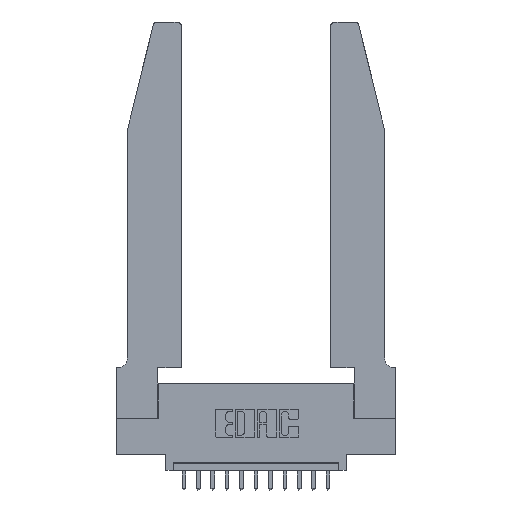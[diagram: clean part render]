
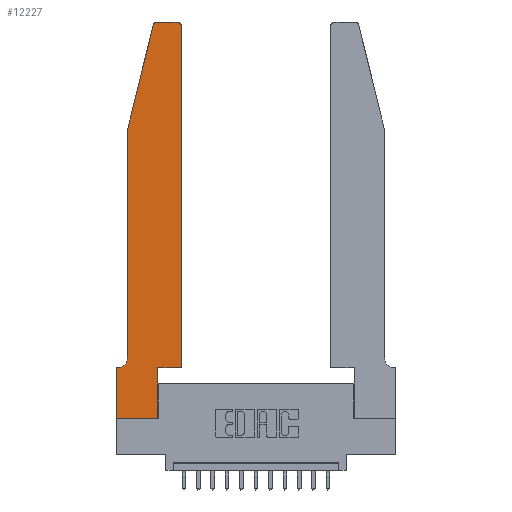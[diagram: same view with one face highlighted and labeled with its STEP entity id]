
A CAD part, top view. The second image highlights one B-rep face of the part: STEP entity #12227.
In plain terms, the highlighted planar face has unit normal (0, 0, 1).
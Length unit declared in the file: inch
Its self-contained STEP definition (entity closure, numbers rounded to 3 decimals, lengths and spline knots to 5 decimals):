
#383 = DIRECTION ( 'NONE',  ( -0.239, -0.971, 0. ) ) ;
#654 = VECTOR ( 'NONE', #7772, 39.37008 ) ;
#697 = VERTEX_POINT ( 'NONE', #13475 ) ;
#800 = EDGE_CURVE ( 'NONE', #697, #3935, #15390, .T. ) ;
#808 = CARTESIAN_POINT ( 'NONE',  ( 0.0755, 2., 0.37 ) ) ;
#819 = CARTESIAN_POINT ( 'NONE',  ( 0., 0., 0.37 ) ) ;
#927 = VERTEX_POINT ( 'NONE', #9903 ) ;
#1074 = VERTEX_POINT ( 'NONE', #10499 ) ;
#1101 = CARTESIAN_POINT ( 'NONE',  ( 0., 0.35, 0.37 ) ) ;
#1359 = AXIS2_PLACEMENT_3D ( 'NONE', #12112, #12005, #14766 ) ;
#1708 = FACE_OUTER_BOUND ( 'NONE', #15711, .T. ) ;
#2040 = EDGE_CURVE ( 'NONE', #9906, #15004, #2591, .T. ) ;
#2212 = DIRECTION ( 'NONE',  ( 1., 0., 0. ) ) ;
#2506 = VERTEX_POINT ( 'NONE', #1101 ) ;
#2591 = LINE ( 'NONE', #808, #11406 ) ;
#2632 = EDGE_CURVE ( 'NONE', #15004, #10120, #17064, .T. ) ;
#2659 = CARTESIAN_POINT ( 'NONE',  ( 0.4205, 2.75, 0.37 ) ) ;
#2793 = ORIENTED_EDGE ( 'NONE', *, *, #10235, .T. ) ;
#2894 = DIRECTION ( 'NONE',  ( 1., 0., 0. ) ) ;
#3178 = LINE ( 'NONE', #12212, #6774 ) ;
#3210 = ORIENTED_EDGE ( 'NONE', *, *, #13313, .T. ) ;
#3414 = CARTESIAN_POINT ( 'NONE',  ( 0.4505, 0.35, 0.37 ) ) ;
#3579 = LINE ( 'NONE', #12251, #6525 ) ;
#3691 = CARTESIAN_POINT ( 'NONE',  ( 0., 0., 0.37 ) ) ;
#3788 = DIRECTION ( 'NONE',  ( 0., 1., 0. ) ) ;
#3935 = VERTEX_POINT ( 'NONE', #2659 ) ;
#4284 = DIRECTION ( 'NONE',  ( 1., 0., 0. ) ) ;
#4287 = EDGE_CURVE ( 'NONE', #927, #14549, #3579, .T. ) ;
#4899 = ORIENTED_EDGE ( 'NONE', *, *, #4287, .T. ) ;
#5090 = VECTOR ( 'NONE', #3788, 39.37008 ) ;
#5359 = CARTESIAN_POINT ( 'NONE',  ( 0.2605, 2.75, 0.37 ) ) ;
#5405 = CIRCLE ( 'NONE', #11653, 0.03 ) ;
#5529 = DIRECTION ( 'NONE',  ( 0., 0., 1. ) ) ;
#5709 = CARTESIAN_POINT ( 'NONE',  ( 0.2865, 0.35, 0.37 ) ) ;
#5763 = VERTEX_POINT ( 'NONE', #10831 ) ;
#6237 = PLANE ( 'NONE',  #8167 ) ;
#6296 = LINE ( 'NONE', #12367, #7558 ) ;
#6525 = VECTOR ( 'NONE', #4284, 39.37008 ) ;
#6668 = CARTESIAN_POINT ( 'NONE',  ( 0., 0., 0.37 ) ) ;
#6716 = DIRECTION ( 'NONE',  ( -1., 0., 0. ) ) ;
#6774 = VECTOR ( 'NONE', #13560, 39.37008 ) ;
#6849 = CARTESIAN_POINT ( 'NONE',  ( 0.0055, 0.35, 0.37 ) ) ;
#6975 = EDGE_CURVE ( 'NONE', #10120, #2506, #3178, .T. ) ;
#6989 = LINE ( 'NONE', #17219, #5090 ) ;
#7034 = EDGE_CURVE ( 'NONE', #9797, #927, #8885, .T. ) ;
#7269 = EDGE_CURVE ( 'NONE', #3935, #5763, #9509, .T. ) ;
#7442 = ORIENTED_EDGE ( 'NONE', *, *, #7994, .T. ) ;
#7473 = CARTESIAN_POINT ( 'NONE',  ( 0.0755, 0.42, 0.37 ) ) ;
#7558 = VECTOR ( 'NONE', #383, 39.37008 ) ;
#7586 = CARTESIAN_POINT ( 'NONE',  ( 0., 0.35, 0.37 ) ) ;
#7772 = DIRECTION ( 'NONE',  ( 0., -1., 0. ) ) ;
#7994 = EDGE_CURVE ( 'NONE', #14549, #697, #6989, .T. ) ;
#8167 = AXIS2_PLACEMENT_3D ( 'NONE', #7586, #16941, #8918 ) ;
#8232 = LINE ( 'NONE', #3691, #654 ) ;
#8383 = VECTOR ( 'NONE', #2894, 39.37008 ) ;
#8885 = LINE ( 'NONE', #5709, #16001 ) ;
#8918 = DIRECTION ( 'NONE',  ( 1., 0., 0. ) ) ;
#9072 = VERTEX_POINT ( 'NONE', #819 ) ;
#9178 = CARTESIAN_POINT ( 'NONE',  ( 0.0755, 2., 0.37 ) ) ;
#9509 = LINE ( 'NONE', #5359, #15366 ) ;
#9797 = VERTEX_POINT ( 'NONE', #11521 ) ;
#9903 = CARTESIAN_POINT ( 'NONE',  ( 0.2865, 0.35, 0.37 ) ) ;
#9906 = VERTEX_POINT ( 'NONE', #9178 ) ;
#10120 = VERTEX_POINT ( 'NONE', #6849 ) ;
#10205 = EDGE_CURVE ( 'NONE', #9072, #9797, #15271, .T. ) ;
#10235 = EDGE_CURVE ( 'NONE', #1074, #9906, #6296, .T. ) ;
#10499 = CARTESIAN_POINT ( 'NONE',  ( 0.25487, 2.72718, 0.37 ) ) ;
#10831 = CARTESIAN_POINT ( 'NONE',  ( 0.284, 2.75, 0.37 ) ) ;
#10977 = ORIENTED_EDGE ( 'NONE', *, *, #800, .T. ) ;
#11406 = VECTOR ( 'NONE', #14574, 39.37008 ) ;
#11521 = CARTESIAN_POINT ( 'NONE',  ( 0.2865, 0., 0.37 ) ) ;
#11653 = AXIS2_PLACEMENT_3D ( 'NONE', #15583, #16950, #2212 ) ;
#12005 = DIRECTION ( 'NONE',  ( 0., 0., -1. ) ) ;
#12112 = CARTESIAN_POINT ( 'NONE',  ( 0.0055, 0.42, 0.37 ) ) ;
#12212 = CARTESIAN_POINT ( 'NONE',  ( 0.0755, 0.35, 0.37 ) ) ;
#12227 = ADVANCED_FACE ( 'NONE', ( #1708 ), #6237, .T. ) ;
#12244 = CARTESIAN_POINT ( 'NONE',  ( 0.4205, 2.72, 0.37 ) ) ;
#12251 = CARTESIAN_POINT ( 'NONE',  ( 0.4505, 0.35, 0.37 ) ) ;
#12367 = CARTESIAN_POINT ( 'NONE',  ( 0.0755, 2., 0.37 ) ) ;
#12573 = ORIENTED_EDGE ( 'NONE', *, *, #7034, .T. ) ;
#13313 = EDGE_CURVE ( 'NONE', #2506, #9072, #8232, .T. ) ;
#13475 = CARTESIAN_POINT ( 'NONE',  ( 0.4505, 2.72, 0.37 ) ) ;
#13525 = DIRECTION ( 'NONE',  ( 0., 1., 0. ) ) ;
#13560 = DIRECTION ( 'NONE',  ( -1., 0., 0. ) ) ;
#13751 = ORIENTED_EDGE ( 'NONE', *, *, #6975, .T. ) ;
#14239 = ORIENTED_EDGE ( 'NONE', *, *, #2040, .T. ) ;
#14549 = VERTEX_POINT ( 'NONE', #3414 ) ;
#14574 = DIRECTION ( 'NONE',  ( 0., -1., 0. ) ) ;
#14766 = DIRECTION ( 'NONE',  ( -1., 0., 0. ) ) ;
#14896 = DIRECTION ( 'NONE',  ( 1., 0., 0. ) ) ;
#14948 = AXIS2_PLACEMENT_3D ( 'NONE', #12244, #5529, #14896 ) ;
#15004 = VERTEX_POINT ( 'NONE', #7473 ) ;
#15204 = ORIENTED_EDGE ( 'NONE', *, *, #7269, .T. ) ;
#15271 = LINE ( 'NONE', #6668, #8383 ) ;
#15366 = VECTOR ( 'NONE', #6716, 39.37008 ) ;
#15390 = CIRCLE ( 'NONE', #14948, 0.03 ) ;
#15565 = ORIENTED_EDGE ( 'NONE', *, *, #16485, .T. ) ;
#15583 = CARTESIAN_POINT ( 'NONE',  ( 0.284, 2.72, 0.37 ) ) ;
#15711 = EDGE_LOOP ( 'NONE', ( #15204, #15565, #2793, #14239, #16958, #13751, #3210, #17299, #12573, #4899, #7442, #10977 ) ) ;
#16001 = VECTOR ( 'NONE', #13525, 39.37008 ) ;
#16485 = EDGE_CURVE ( 'NONE', #5763, #1074, #5405, .T. ) ;
#16941 = DIRECTION ( 'NONE',  ( 0., 0., 1. ) ) ;
#16950 = DIRECTION ( 'NONE',  ( 0., 0., 1. ) ) ;
#16958 = ORIENTED_EDGE ( 'NONE', *, *, #2632, .T. ) ;
#17064 = CIRCLE ( 'NONE', #1359, 0.07 ) ;
#17219 = CARTESIAN_POINT ( 'NONE',  ( 0.4505, 0.35, 0.37 ) ) ;
#17299 = ORIENTED_EDGE ( 'NONE', *, *, #10205, .T. ) ;
